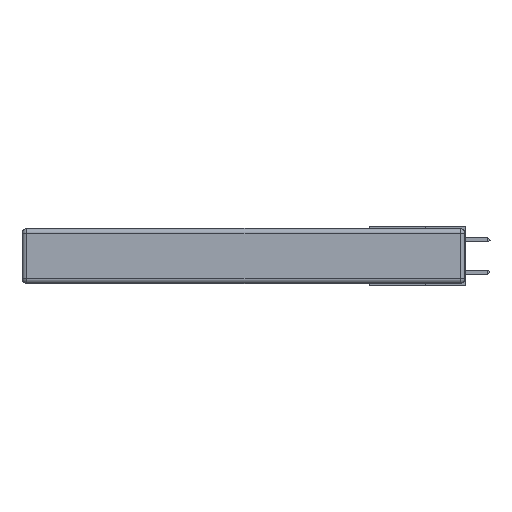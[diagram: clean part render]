
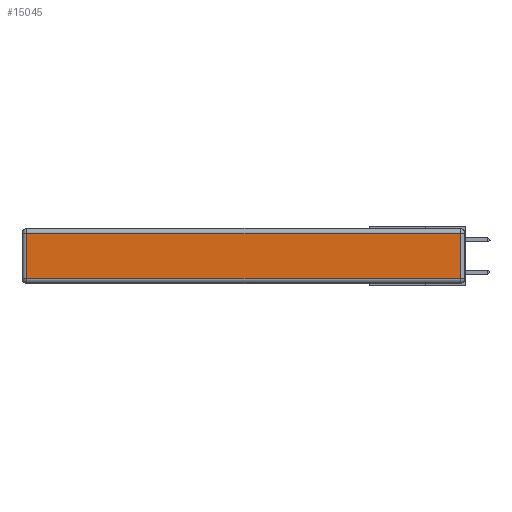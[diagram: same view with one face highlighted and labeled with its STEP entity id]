
A CAD part, left-side view. The second image highlights one B-rep face of the part: STEP entity #15045.
In plain terms, the highlighted planar face has unit normal (-1, 0, 0).
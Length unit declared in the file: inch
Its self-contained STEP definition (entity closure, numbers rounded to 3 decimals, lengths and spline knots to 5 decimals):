
#535 = EDGE_LOOP ( 'NONE', ( #15695, #29539, #15702, #3329 ) ) ;
#784 = CARTESIAN_POINT ( 'NONE',  ( 0., 2.72, -0.313 ) ) ;
#1456 = CARTESIAN_POINT ( 'NONE',  ( 0., 2.75, -0.03 ) ) ;
#1469 = EDGE_CURVE ( 'NONE', #15235, #19604, #20135, .T. ) ;
#2078 = AXIS2_PLACEMENT_3D ( 'NONE', #3822, #19542, #26496 ) ;
#3054 = VERTEX_POINT ( 'NONE', #29097 ) ;
#3329 = ORIENTED_EDGE ( 'NONE', *, *, #3919, .T. ) ;
#3822 = CARTESIAN_POINT ( 'NONE',  ( 0., 0., -0.343 ) ) ;
#3919 = EDGE_CURVE ( 'NONE', #3054, #23131, #7096, .T. ) ;
#7096 = LINE ( 'NONE', #12672, #22143 ) ;
#8152 = EDGE_CURVE ( 'NONE', #19604, #3054, #22857, .T. ) ;
#8772 = VECTOR ( 'NONE', #25696, 39.37008 ) ;
#8920 = VECTOR ( 'NONE', #19849, 39.37008 ) ;
#9223 = CARTESIAN_POINT ( 'NONE',  ( 0., 0.03, -0.313 ) ) ;
#9475 = LINE ( 'NONE', #14470, #8772 ) ;
#10527 = PLANE ( 'NONE',  #2078 ) ;
#12324 = FACE_OUTER_BOUND ( 'NONE', #535, .T. ) ;
#12672 = CARTESIAN_POINT ( 'NONE',  ( 0., 2.72, -0.343 ) ) ;
#14058 = VECTOR ( 'NONE', #18568, 39.37008 ) ;
#14470 = CARTESIAN_POINT ( 'NONE',  ( 0., 0., -0.313 ) ) ;
#14992 = DIRECTION ( 'NONE',  ( 0., 0., -1. ) ) ;
#15045 = ADVANCED_FACE ( 'NONE', ( #12324 ), #10527, .T. ) ;
#15235 = VERTEX_POINT ( 'NONE', #9223 ) ;
#15695 = ORIENTED_EDGE ( 'NONE', *, *, #22090, .T. ) ;
#15702 = ORIENTED_EDGE ( 'NONE', *, *, #8152, .T. ) ;
#18568 = DIRECTION ( 'NONE',  ( 0., 0., 1. ) ) ;
#19542 = DIRECTION ( 'NONE',  ( -1., 0., 0. ) ) ;
#19604 = VERTEX_POINT ( 'NONE', #25136 ) ;
#19849 = DIRECTION ( 'NONE',  ( 0., 1., 0. ) ) ;
#20135 = LINE ( 'NONE', #27407, #14058 ) ;
#22090 = EDGE_CURVE ( 'NONE', #23131, #15235, #9475, .T. ) ;
#22143 = VECTOR ( 'NONE', #14992, 39.37008 ) ;
#22857 = LINE ( 'NONE', #1456, #8920 ) ;
#23131 = VERTEX_POINT ( 'NONE', #784 ) ;
#25136 = CARTESIAN_POINT ( 'NONE',  ( 0., 0.03, -0.03 ) ) ;
#25696 = DIRECTION ( 'NONE',  ( 0., -1., 0. ) ) ;
#26496 = DIRECTION ( 'NONE',  ( 0., 0., 1. ) ) ;
#27407 = CARTESIAN_POINT ( 'NONE',  ( 0., 0.03, -0.343 ) ) ;
#29097 = CARTESIAN_POINT ( 'NONE',  ( 0., 2.72, -0.03 ) ) ;
#29539 = ORIENTED_EDGE ( 'NONE', *, *, #1469, .T. ) ;
